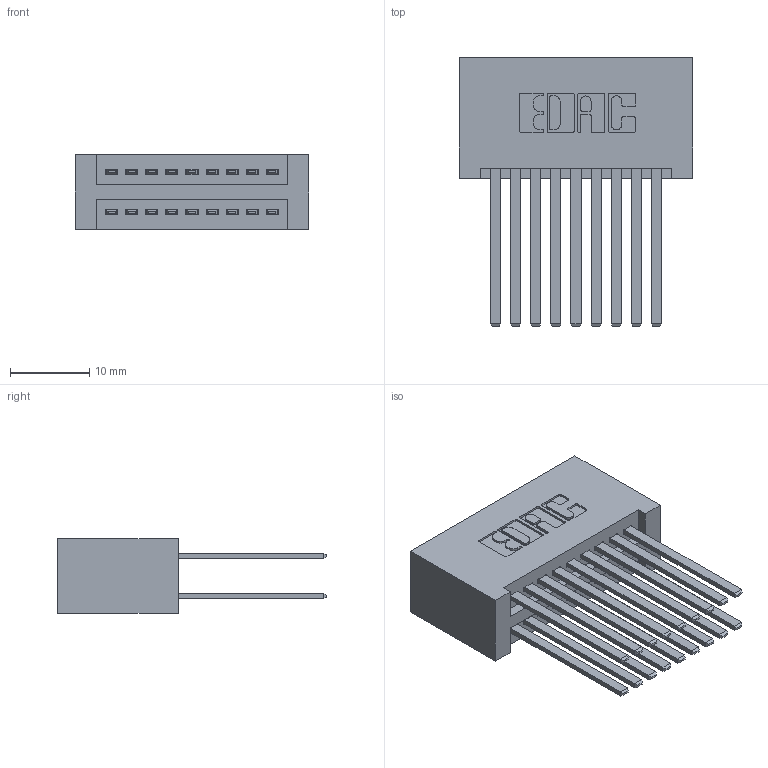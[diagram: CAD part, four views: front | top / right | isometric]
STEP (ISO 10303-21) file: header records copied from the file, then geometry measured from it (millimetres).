
FILE_DESCRIPTION (( 'STEP AP203' ), '1' );
FILE_NAME ('395-018-544-201.STEP', '2018-11-07T02:46:47', ( '' ), ( '' ), 'SwSTEP 2.0', 'SolidWorks 2016', '' );
FILE_SCHEMA (( 'CONFIG_CONTROL_DESIGN' ));
Length unit declared in the file: inch
Products named in the file (3): 395-018-544-201; 345-292-001_345-293-144; 345 Part_No Mounting Lugs
Assembly tree (19 placements, depth 2):
  395-018-544-201
    345 Part_No Mounting Lugs
    345-292-001_345-293-144  x18
Bounding box: 29.46 x 33.96 x 9.4 mm (x, y, z)
Volume: 3424.1 mm3; surface area: 5465 mm2
Topology: 19 solids, 19 shells, 910 faces, 2675 edges, 1758 vertices
Faces by surface type: plane 598, cylinder 312
Entity records: 11043 total; most frequent: CARTESIAN_POINT 1880, ORIENTED_EDGE 1814, DIRECTION 1691, EDGE_CURVE 907, LINE 751, VECTOR 751, VERTEX_POINT 602, AXIS2_PLACEMENT_3D 470
